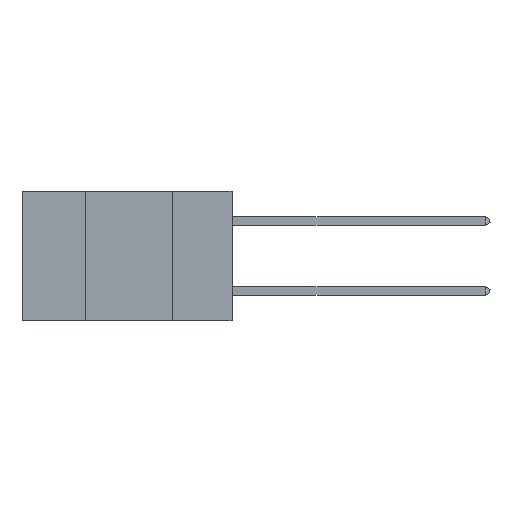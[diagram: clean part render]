
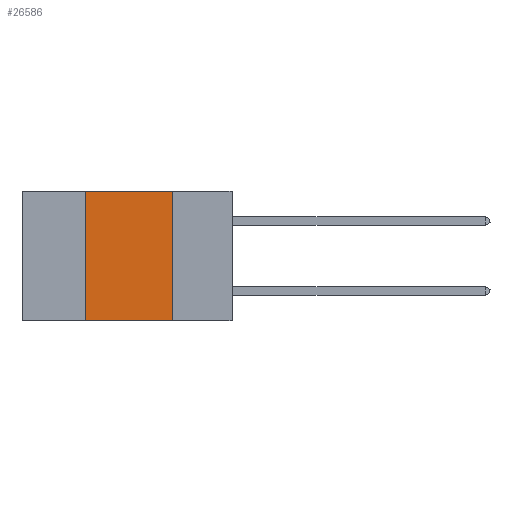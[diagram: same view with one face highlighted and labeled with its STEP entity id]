
A CAD part, left-side view. The second image highlights one B-rep face of the part: STEP entity #26586.
In plain terms, the highlighted planar face has unit normal (-1, 0, 0).
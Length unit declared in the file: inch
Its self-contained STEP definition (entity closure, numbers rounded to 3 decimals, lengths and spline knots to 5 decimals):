
#240 = EDGE_CURVE ( 'NONE', #35187, #27984, #44706, .T. ) ;
#854 = ORIENTED_EDGE ( 'NONE', *, *, #7251, .F. ) ;
#2687 = CARTESIAN_POINT ( 'NONE',  ( 0., 0.6, 0. ) ) ;
#7251 = EDGE_CURVE ( 'NONE', #10794, #35187, #35458, .T. ) ;
#9942 = AXIS2_PLACEMENT_3D ( 'NONE', #10132, #31914, #45667 ) ;
#10132 = CARTESIAN_POINT ( 'NONE',  ( 0., 0.6, 0. ) ) ;
#10794 = VERTEX_POINT ( 'NONE', #24149 ) ;
#10940 = LINE ( 'NONE', #25483, #27140 ) ;
#12341 = ORIENTED_EDGE ( 'NONE', *, *, #14356, .T. ) ;
#13717 = CARTESIAN_POINT ( 'NONE',  ( 0., 0.17, -0.37 ) ) ;
#14356 = EDGE_CURVE ( 'NONE', #15205, #27984, #10940, .T. ) ;
#15205 = VERTEX_POINT ( 'NONE', #41239 ) ;
#18086 = CARTESIAN_POINT ( 'NONE',  ( 0., 0.17, 0. ) ) ;
#18742 = CARTESIAN_POINT ( 'NONE',  ( 0., 0.42, 0. ) ) ;
#19208 = ORIENTED_EDGE ( 'NONE', *, *, #240, .F. ) ;
#20399 = VECTOR ( 'NONE', #29800, 39.37008 ) ;
#23331 = EDGE_LOOP ( 'NONE', ( #19208, #854, #39509, #12341 ) ) ;
#24149 = CARTESIAN_POINT ( 'NONE',  ( 0., 0.42, 0. ) ) ;
#25483 = CARTESIAN_POINT ( 'NONE',  ( 0., 0.6, -0.37 ) ) ;
#26586 = ADVANCED_FACE ( 'NONE', ( #37440 ), #42200, .F. ) ;
#26926 = DIRECTION ( 'NONE',  ( 0., 0., -1. ) ) ;
#27140 = VECTOR ( 'NONE', #29061, 39.37008 ) ;
#27984 = VERTEX_POINT ( 'NONE', #13717 ) ;
#29061 = DIRECTION ( 'NONE',  ( 0., -1., 0. ) ) ;
#29597 = VECTOR ( 'NONE', #26926, 39.37008 ) ;
#29800 = DIRECTION ( 'NONE',  ( 0., 0., 1. ) ) ;
#31914 = DIRECTION ( 'NONE',  ( 1., 0., 0. ) ) ;
#32100 = VECTOR ( 'NONE', #38470, 39.37008 ) ;
#34367 = CARTESIAN_POINT ( 'NONE',  ( 0., 0.17, 0. ) ) ;
#35187 = VERTEX_POINT ( 'NONE', #18086 ) ;
#35458 = LINE ( 'NONE', #2687, #32100 ) ;
#37440 = FACE_OUTER_BOUND ( 'NONE', #23331, .T. ) ;
#38470 = DIRECTION ( 'NONE',  ( 0., -1., 0. ) ) ;
#39363 = LINE ( 'NONE', #18742, #20399 ) ;
#39509 = ORIENTED_EDGE ( 'NONE', *, *, #44880, .F. ) ;
#41239 = CARTESIAN_POINT ( 'NONE',  ( 0., 0.42, -0.37 ) ) ;
#42200 = PLANE ( 'NONE',  #9942 ) ;
#44706 = LINE ( 'NONE', #34367, #29597 ) ;
#44880 = EDGE_CURVE ( 'NONE', #15205, #10794, #39363, .T. ) ;
#45667 = DIRECTION ( 'NONE',  ( 0., 0., -1. ) ) ;
